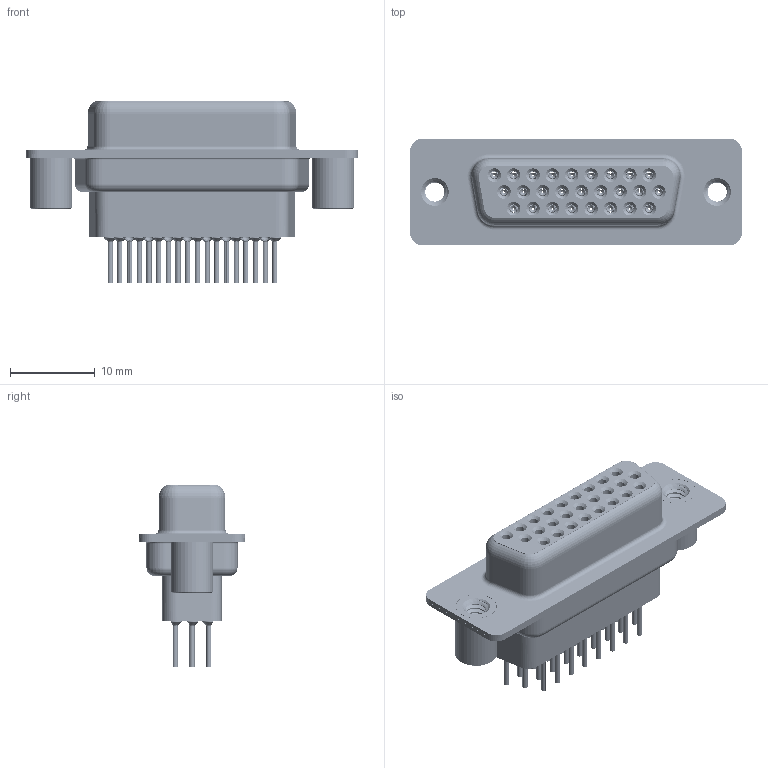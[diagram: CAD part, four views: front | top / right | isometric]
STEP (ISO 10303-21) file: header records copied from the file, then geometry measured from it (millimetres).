
FILE_DESCRIPTION (( 'STEP AP203' ), '1' );
FILE_NAME ('638-026-231-259.STEP', '2020-07-18T19:57:33', ( '' ), ( '' ), 'SwSTEP 2.0', 'SolidWorks 2020', '' );
FILE_SCHEMA (( 'CONFIG_CONTROL_DESIGN' ));
Length unit declared in the file: millimetre
Products named in the file (8): 638 Shell Rear_26 Contacts; 638-026-231-259; 638 Shell Front_26 Contacts; 638 Housing_26 Contacts HP; 638 Contact Row 3_31; 638 4-40 Threaded Standoff BS; 638 Contact Row 1_31; 638 Contact Row 2_31
Assembly tree (31 placements, depth 2):
  638-026-231-259
    638 Housing_26 Contacts HP
    638 Shell Front_26 Contacts
    638 Shell Rear_26 Contacts
    638 Contact Row 1_31  x9
    638 Contact Row 2_31  x9
    638 Contact Row 3_31  x8
    638 4-40 Threaded Standoff BS  x2
Bounding box: 39.19 x 12.6 x 21.5 mm (x, y, z)
Volume: 2772.3 mm3; surface area: 10061.3 mm2
Topology: 31 solids, 31 shells, 3499 faces, 8965 edges, 5591 vertices
Faces by surface type: cylinder 1015, plane 873, torus 681, bspline 526, cone 404
Entity records: 33173 total; most frequent: CARTESIAN_POINT 10043, DIRECTION 4689, ORIENTED_EDGE 4450, EDGE_CURVE 2225, AXIS2_PLACEMENT_3D 1956, VERTEX_POINT 1401, EDGE_LOOP 1078, CIRCLE 1060
